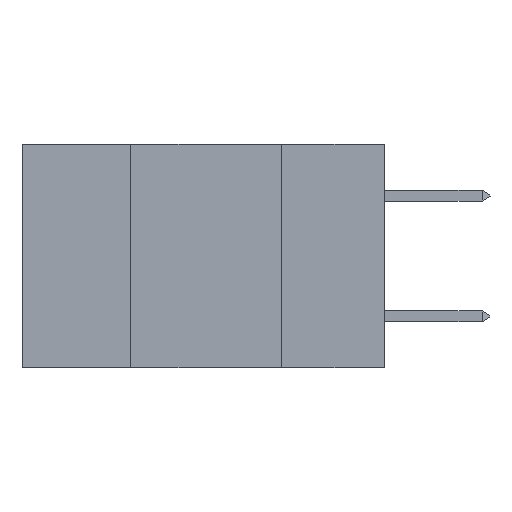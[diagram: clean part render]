
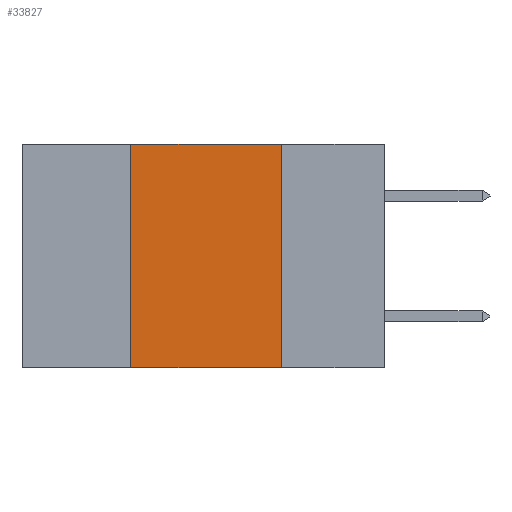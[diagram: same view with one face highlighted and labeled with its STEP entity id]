
A CAD part, left-side view. The second image highlights one B-rep face of the part: STEP entity #33827.
In plain terms, the highlighted planar face has unit normal (-1, 0, 0).
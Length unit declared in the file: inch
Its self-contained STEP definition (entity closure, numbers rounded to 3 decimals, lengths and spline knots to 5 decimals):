
#517 = VERTEX_POINT ( 'NONE', #16678 ) ;
#1391 = DIRECTION ( 'NONE',  ( 0., -1., 0. ) ) ;
#2562 = FACE_OUTER_BOUND ( 'NONE', #19017, .T. ) ;
#3066 = AXIS2_PLACEMENT_3D ( 'NONE', #24902, #26894, #30814 ) ;
#4191 = CARTESIAN_POINT ( 'NONE',  ( 0., 0.42, 0. ) ) ;
#8438 = CARTESIAN_POINT ( 'NONE',  ( 0., 0.6, -0.37 ) ) ;
#9177 = EDGE_CURVE ( 'NONE', #31221, #29716, #16097, .T. ) ;
#10618 = ORIENTED_EDGE ( 'NONE', *, *, #21177, .F. ) ;
#11600 = LINE ( 'NONE', #33586, #18370 ) ;
#12775 = VECTOR ( 'NONE', #19904, 39.37008 ) ;
#13886 = PLANE ( 'NONE',  #3066 ) ;
#14367 = CARTESIAN_POINT ( 'NONE',  ( 0., 0.42, -0.37 ) ) ;
#16097 = LINE ( 'NONE', #32485, #29325 ) ;
#16678 = CARTESIAN_POINT ( 'NONE',  ( 0., 0.17, 0. ) ) ;
#18131 = EDGE_CURVE ( 'NONE', #517, #23305, #11600, .T. ) ;
#18370 = VECTOR ( 'NONE', #27841, 39.37008 ) ;
#19017 = EDGE_LOOP ( 'NONE', ( #23040, #10618, #26950, #24341 ) ) ;
#19904 = DIRECTION ( 'NONE',  ( 0., -1., 0. ) ) ;
#20764 = EDGE_CURVE ( 'NONE', #31221, #23305, #33099, .T. ) ;
#21177 = EDGE_CURVE ( 'NONE', #29716, #517, #34311, .T. ) ;
#23040 = ORIENTED_EDGE ( 'NONE', *, *, #18131, .F. ) ;
#23226 = CARTESIAN_POINT ( 'NONE',  ( 0., 0.17, -0.37 ) ) ;
#23305 = VERTEX_POINT ( 'NONE', #23226 ) ;
#24341 = ORIENTED_EDGE ( 'NONE', *, *, #20764, .T. ) ;
#24902 = CARTESIAN_POINT ( 'NONE',  ( 0., 0.6, 0. ) ) ;
#25427 = VECTOR ( 'NONE', #1391, 39.37008 ) ;
#26894 = DIRECTION ( 'NONE',  ( 1., 0., 0. ) ) ;
#26950 = ORIENTED_EDGE ( 'NONE', *, *, #9177, .F. ) ;
#27841 = DIRECTION ( 'NONE',  ( 0., 0., -1. ) ) ;
#29259 = DIRECTION ( 'NONE',  ( 0., 0., 1. ) ) ;
#29325 = VECTOR ( 'NONE', #29259, 39.37008 ) ;
#29716 = VERTEX_POINT ( 'NONE', #4191 ) ;
#30814 = DIRECTION ( 'NONE',  ( 0., 0., -1. ) ) ;
#30889 = CARTESIAN_POINT ( 'NONE',  ( 0., 0.6, 0. ) ) ;
#31221 = VERTEX_POINT ( 'NONE', #14367 ) ;
#32485 = CARTESIAN_POINT ( 'NONE',  ( 0., 0.42, 0. ) ) ;
#33099 = LINE ( 'NONE', #8438, #25427 ) ;
#33586 = CARTESIAN_POINT ( 'NONE',  ( 0., 0.17, 0. ) ) ;
#33827 = ADVANCED_FACE ( 'NONE', ( #2562 ), #13886, .F. ) ;
#34311 = LINE ( 'NONE', #30889, #12775 ) ;
